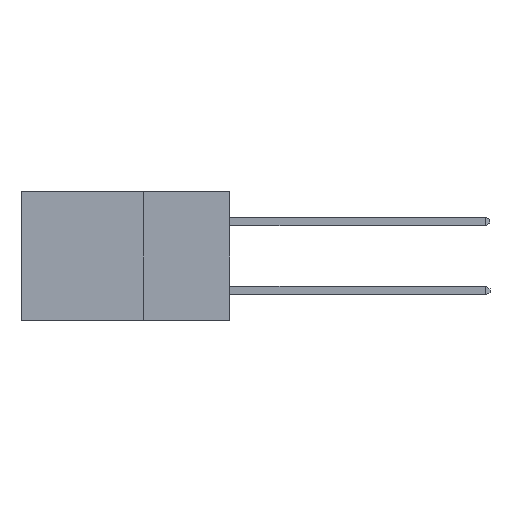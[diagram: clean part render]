
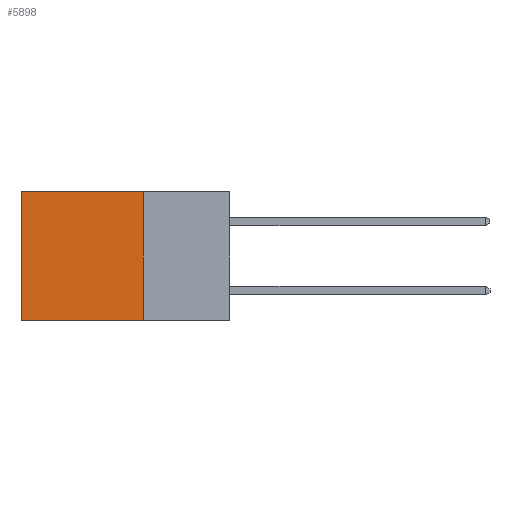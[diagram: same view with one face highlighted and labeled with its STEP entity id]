
A CAD part, left-side view. The second image highlights one B-rep face of the part: STEP entity #5898.
In plain terms, the highlighted planar face has unit normal (-1, 0, 0).
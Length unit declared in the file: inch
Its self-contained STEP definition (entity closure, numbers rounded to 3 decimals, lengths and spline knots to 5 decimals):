
#247 = VERTEX_POINT ( 'NONE', #10491 ) ;
#423 = LINE ( 'NONE', #4528, #5385 ) ;
#846 = FACE_OUTER_BOUND ( 'NONE', #11161, .T. ) ;
#1041 = VERTEX_POINT ( 'NONE', #10012 ) ;
#1633 = LINE ( 'NONE', #2396, #3893 ) ;
#2283 = DIRECTION ( 'NONE',  ( 0., 0., -1. ) ) ;
#2396 = CARTESIAN_POINT ( 'NONE',  ( 0.2615, 0.6, -0.37 ) ) ;
#2990 = EDGE_CURVE ( 'NONE', #247, #10756, #5853, .T. ) ;
#3797 = DIRECTION ( 'NONE',  ( 0., 0., -1. ) ) ;
#3808 = CARTESIAN_POINT ( 'NONE',  ( 0.2615, 0.25, -0.37 ) ) ;
#3893 = VECTOR ( 'NONE', #2283, 39.37008 ) ;
#4528 = CARTESIAN_POINT ( 'NONE',  ( 0.2615, 0.25, 0. ) ) ;
#4870 = ORIENTED_EDGE ( 'NONE', *, *, #5395, .F. ) ;
#5225 = VERTEX_POINT ( 'NONE', #5913 ) ;
#5385 = VECTOR ( 'NONE', #5786, 39.37008 ) ;
#5395 = EDGE_CURVE ( 'NONE', #10756, #1041, #11705, .T. ) ;
#5786 = DIRECTION ( 'NONE',  ( 0., 1., 0. ) ) ;
#5853 = LINE ( 'NONE', #3808, #10937 ) ;
#5896 = CARTESIAN_POINT ( 'NONE',  ( 0.2615, 0.25, -0.37 ) ) ;
#5898 = ADVANCED_FACE ( 'NONE', ( #846 ), #12444, .F. ) ;
#5913 = CARTESIAN_POINT ( 'NONE',  ( 0.2615, 0.6, 0. ) ) ;
#5959 = DIRECTION ( 'NONE',  ( 0., 1., 0. ) ) ;
#6380 = CARTESIAN_POINT ( 'NONE',  ( 0.2615, 0.25, -0.37 ) ) ;
#6573 = ORIENTED_EDGE ( 'NONE', *, *, #6593, .T. ) ;
#6593 = EDGE_CURVE ( 'NONE', #5225, #1041, #1633, .T. ) ;
#7011 = VECTOR ( 'NONE', #5959, 39.37008 ) ;
#8745 = EDGE_CURVE ( 'NONE', #247, #5225, #423, .T. ) ;
#9213 = ORIENTED_EDGE ( 'NONE', *, *, #8745, .T. ) ;
#10012 = CARTESIAN_POINT ( 'NONE',  ( 0.2615, 0.6, -0.37 ) ) ;
#10108 = ORIENTED_EDGE ( 'NONE', *, *, #2990, .F. ) ;
#10491 = CARTESIAN_POINT ( 'NONE',  ( 0.2615, 0.25, 0. ) ) ;
#10756 = VERTEX_POINT ( 'NONE', #6380 ) ;
#10774 = AXIS2_PLACEMENT_3D ( 'NONE', #12218, #12171, #12154 ) ;
#10937 = VECTOR ( 'NONE', #3797, 39.37008 ) ;
#11161 = EDGE_LOOP ( 'NONE', ( #6573, #4870, #10108, #9213 ) ) ;
#11705 = LINE ( 'NONE', #5896, #7011 ) ;
#12154 = DIRECTION ( 'NONE',  ( 0., 0., -1. ) ) ;
#12171 = DIRECTION ( 'NONE',  ( 1., 0., 0. ) ) ;
#12218 = CARTESIAN_POINT ( 'NONE',  ( 0.2615, 0.25, -0.37 ) ) ;
#12444 = PLANE ( 'NONE',  #10774 ) ;
